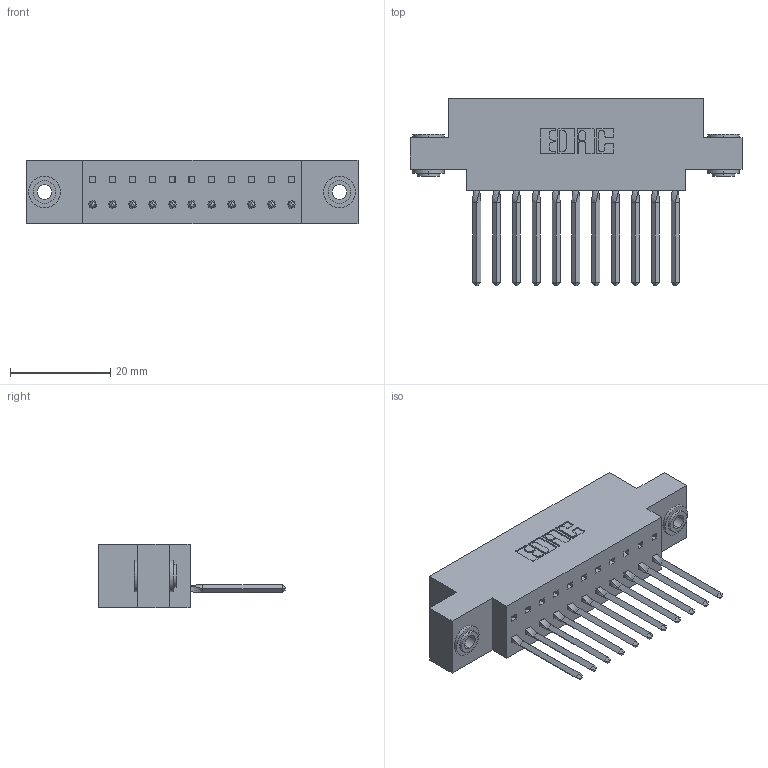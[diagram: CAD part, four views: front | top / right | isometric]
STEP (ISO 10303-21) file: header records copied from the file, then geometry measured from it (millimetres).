
FILE_DESCRIPTION (( 'STEP AP203' ), '1' );
FILE_NAME ('317-011-541-603.STEP', '2020-02-27T13:46:01', ( '' ), ( '' ), 'SwSTEP 2.0', 'SolidWorks 2016', '' );
FILE_SCHEMA (( 'CONFIG_CONTROL_DESIGN' ));
Length unit declared in the file: inch
Products named in the file (4): 317-011-541-603; 317-290-002_541; 317 Part_.156 Dia - TH; 345-250-002_345-250-002-102
Assembly tree (14 placements, depth 2):
  317-011-541-603
    317 Part_.156 Dia - TH
    317-290-002_541  x11
    345-250-002_345-250-002-102  x2
Bounding box: 66.29 x 37.34 x 12.7 mm (x, y, z)
Volume: 9816.9 mm3; surface area: 13053 mm2
Topology: 14 solids, 14 shells, 1812 faces, 5125 edges, 3332 vertices
Faces by surface type: plane 1432, cylinder 328, bspline 44, cone 8
Entity records: 22071 total; most frequent: CARTESIAN_POINT 4517, ORIENTED_EDGE 3774, DIRECTION 3119, EDGE_CURVE 1887, LINE 1499, VECTOR 1499, VERTEX_POINT 1248, AXIS2_PLACEMENT_3D 810
